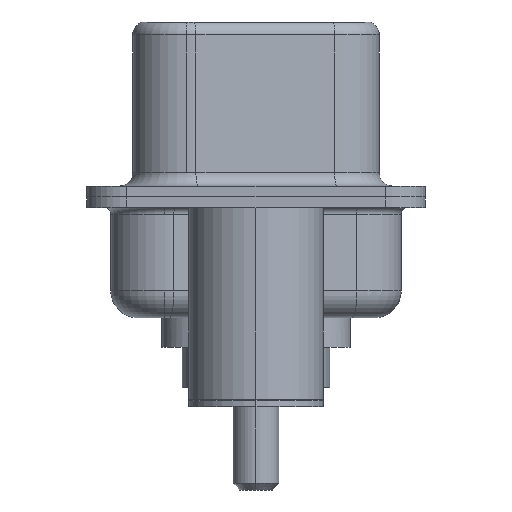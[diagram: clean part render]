
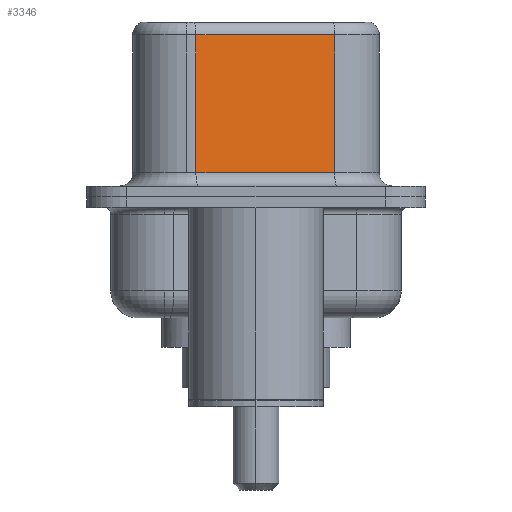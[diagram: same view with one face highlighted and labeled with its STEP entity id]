
A CAD part, left-side view. The second image highlights one B-rep face of the part: STEP entity #3346.
In plain terms, the highlighted planar face has unit normal (-0.985, -0.174, 0).
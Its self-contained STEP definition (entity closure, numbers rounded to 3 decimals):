
#232 = DIRECTION ( 'NONE',  ( -0.174, 0.985, 0. ) ) ;
#237 = DIRECTION ( 'NONE',  ( 0.985, 0.174, 0. ) ) ;
#250 = PLANE ( 'NONE',  #10517 ) ;
#410 = EDGE_CURVE ( 'NONE', #2490, #4172, #6073, .T. ) ;
#435 = CARTESIAN_POINT ( 'NONE',  ( 3.67, 2.233, 6.02 ) ) ;
#866 = CARTESIAN_POINT ( 'NONE',  ( 4.58, -2.927, 6.02 ) ) ;
#1150 = EDGE_CURVE ( 'NONE', #13152, #4172, #1409, .T. ) ;
#1359 = CARTESIAN_POINT ( 'NONE',  ( 3.67, 2.233, 6.52 ) ) ;
#1409 = LINE ( 'NONE', #8382, #4910 ) ;
#1457 = CARTESIAN_POINT ( 'NONE',  ( 4.58, -2.927, 6.52 ) ) ;
#2369 = EDGE_LOOP ( 'NONE', ( #8941, #7903, #11708, #2689 ) ) ;
#2490 = VERTEX_POINT ( 'NONE', #5389 ) ;
#2689 = ORIENTED_EDGE ( 'NONE', *, *, #410, .T. ) ;
#2970 = EDGE_CURVE ( 'NONE', #9161, #2490, #11434, .T. ) ;
#3253 = DIRECTION ( 'NONE',  ( 0., 0., -1. ) ) ;
#3346 = ADVANCED_FACE ( 'NONE', ( #7206 ), #250, .F. ) ;
#4172 = VERTEX_POINT ( 'NONE', #14743 ) ;
#4542 = DIRECTION ( 'NONE',  ( 0., 0., -1. ) ) ;
#4910 = VECTOR ( 'NONE', #4542, 1000. ) ;
#5167 = EDGE_CURVE ( 'NONE', #13152, #9161, #14751, .T. ) ;
#5389 = CARTESIAN_POINT ( 'NONE',  ( 3.67, 2.233, 0.9 ) ) ;
#5394 = VECTOR ( 'NONE', #12710, 1000. ) ;
#6073 = LINE ( 'NONE', #14044, #11668 ) ;
#7206 = FACE_OUTER_BOUND ( 'NONE', #2369, .T. ) ;
#7903 = ORIENTED_EDGE ( 'NONE', *, *, #5167, .T. ) ;
#8152 = VECTOR ( 'NONE', #3253, 1000. ) ;
#8382 = CARTESIAN_POINT ( 'NONE',  ( 4.58, -2.927, 6.52 ) ) ;
#8941 = ORIENTED_EDGE ( 'NONE', *, *, #1150, .F. ) ;
#9161 = VERTEX_POINT ( 'NONE', #435 ) ;
#10517 = AXIS2_PLACEMENT_3D ( 'NONE', #1457, #237, #232 ) ;
#11434 = LINE ( 'NONE', #1359, #8152 ) ;
#11668 = VECTOR ( 'NONE', #13897, 1000. ) ;
#11708 = ORIENTED_EDGE ( 'NONE', *, *, #2970, .T. ) ;
#12710 = DIRECTION ( 'NONE',  ( -0.174, 0.985, 0. ) ) ;
#13152 = VERTEX_POINT ( 'NONE', #866 ) ;
#13255 = CARTESIAN_POINT ( 'NONE',  ( 4.58, -2.927, 6.02 ) ) ;
#13897 = DIRECTION ( 'NONE',  ( 0.174, -0.985, 0. ) ) ;
#14044 = CARTESIAN_POINT ( 'NONE',  ( 4.58, -2.927, 0.9 ) ) ;
#14743 = CARTESIAN_POINT ( 'NONE',  ( 4.58, -2.927, 0.9 ) ) ;
#14751 = LINE ( 'NONE', #13255, #5394 ) ;
